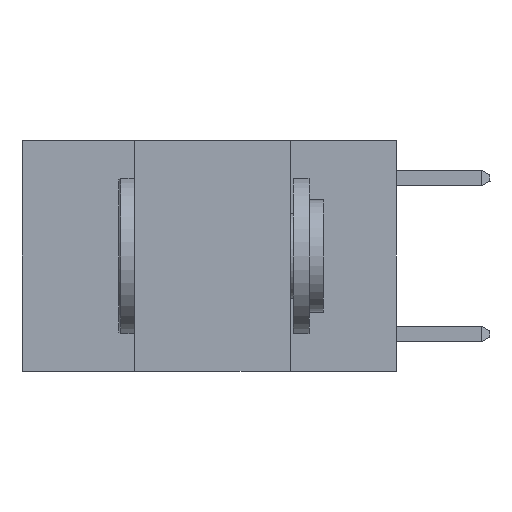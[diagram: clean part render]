
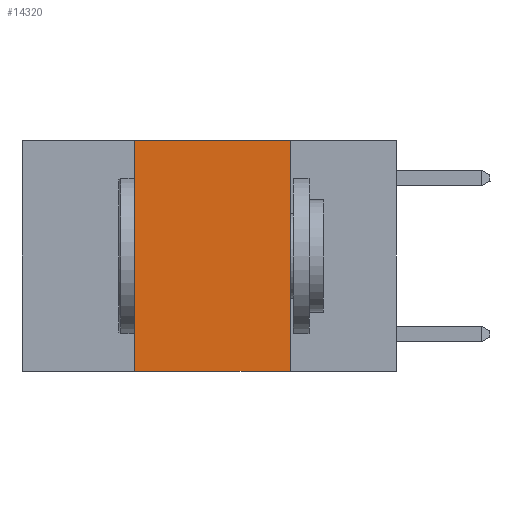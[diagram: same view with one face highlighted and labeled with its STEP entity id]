
A CAD part, left-side view. The second image highlights one B-rep face of the part: STEP entity #14320.
In plain terms, the highlighted planar face has unit normal (-1, 0, 0).
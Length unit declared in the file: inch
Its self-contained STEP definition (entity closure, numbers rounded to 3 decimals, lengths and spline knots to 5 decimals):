
#14 = PLANE ( 'NONE',  #9081 ) ;
#106 = DIRECTION ( 'NONE',  ( 0., 0., -1. ) ) ;
#801 = LINE ( 'NONE', #986, #7545 ) ;
#985 = EDGE_CURVE ( 'NONE', #8901, #14423, #801, .T. ) ;
#986 = CARTESIAN_POINT ( 'NONE',  ( 0., 0.6, 0. ) ) ;
#1460 = DIRECTION ( 'NONE',  ( 1., 0., 0. ) ) ;
#1765 = EDGE_CURVE ( 'NONE', #1835, #16550, #3876, .T. ) ;
#1767 = CARTESIAN_POINT ( 'NONE',  ( 0., 0.42, -0.37 ) ) ;
#1835 = VERTEX_POINT ( 'NONE', #1767 ) ;
#3839 = VECTOR ( 'NONE', #15436, 39.37008 ) ;
#3876 = LINE ( 'NONE', #8093, #10969 ) ;
#3985 = EDGE_CURVE ( 'NONE', #14423, #16550, #5635, .T. ) ;
#4644 = EDGE_LOOP ( 'NONE', ( #4788, #5324, #9354, #11844 ) ) ;
#4788 = ORIENTED_EDGE ( 'NONE', *, *, #3985, .F. ) ;
#5160 = EDGE_CURVE ( 'NONE', #1835, #8901, #13829, .T. ) ;
#5324 = ORIENTED_EDGE ( 'NONE', *, *, #985, .F. ) ;
#5635 = LINE ( 'NONE', #11107, #3839 ) ;
#7545 = VECTOR ( 'NONE', #7756, 39.37008 ) ;
#7756 = DIRECTION ( 'NONE',  ( 0., -1., 0. ) ) ;
#8093 = CARTESIAN_POINT ( 'NONE',  ( 0., 0.6, -0.37 ) ) ;
#8438 = CARTESIAN_POINT ( 'NONE',  ( 0., 0.17, -0.37 ) ) ;
#8487 = VECTOR ( 'NONE', #13999, 39.37008 ) ;
#8901 = VERTEX_POINT ( 'NONE', #10555 ) ;
#9081 = AXIS2_PLACEMENT_3D ( 'NONE', #13808, #1460, #106 ) ;
#9354 = ORIENTED_EDGE ( 'NONE', *, *, #5160, .F. ) ;
#10555 = CARTESIAN_POINT ( 'NONE',  ( 0., 0.42, 0. ) ) ;
#10969 = VECTOR ( 'NONE', #14935, 39.37008 ) ;
#11107 = CARTESIAN_POINT ( 'NONE',  ( 0., 0.17, 0. ) ) ;
#11215 = CARTESIAN_POINT ( 'NONE',  ( 0., 0.42, 0. ) ) ;
#11844 = ORIENTED_EDGE ( 'NONE', *, *, #1765, .T. ) ;
#12985 = CARTESIAN_POINT ( 'NONE',  ( 0., 0.17, 0. ) ) ;
#13808 = CARTESIAN_POINT ( 'NONE',  ( 0., 0.6, 0. ) ) ;
#13829 = LINE ( 'NONE', #11215, #8487 ) ;
#13999 = DIRECTION ( 'NONE',  ( 0., 0., 1. ) ) ;
#14320 = ADVANCED_FACE ( 'NONE', ( #16417 ), #14, .F. ) ;
#14423 = VERTEX_POINT ( 'NONE', #12985 ) ;
#14935 = DIRECTION ( 'NONE',  ( 0., -1., 0. ) ) ;
#15436 = DIRECTION ( 'NONE',  ( 0., 0., -1. ) ) ;
#16417 = FACE_OUTER_BOUND ( 'NONE', #4644, .T. ) ;
#16550 = VERTEX_POINT ( 'NONE', #8438 ) ;
